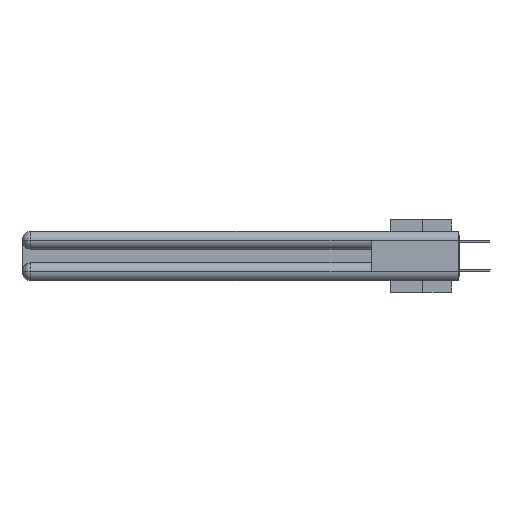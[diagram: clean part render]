
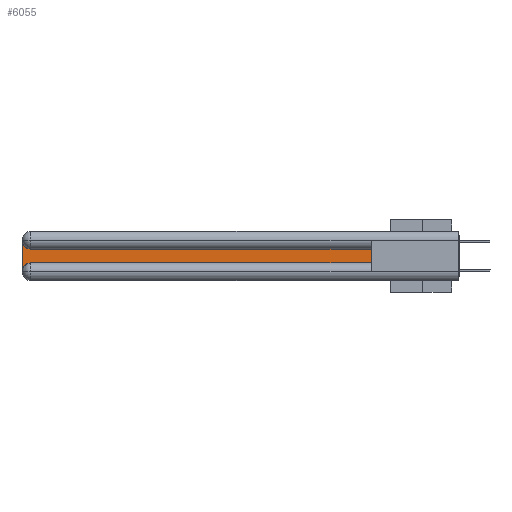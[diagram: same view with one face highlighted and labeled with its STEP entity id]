
A CAD part, left-side view. The second image highlights one B-rep face of the part: STEP entity #6055.
In plain terms, the highlighted planar face has unit normal (-1, 0, 0).
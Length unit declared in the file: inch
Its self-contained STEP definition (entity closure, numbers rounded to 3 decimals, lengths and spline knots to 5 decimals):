
#115 = CARTESIAN_POINT ( 'NONE',  ( 0.075, 3., -0.1225 ) ) ;
#227 = CIRCLE ( 'NONE', #17963, 0.06 ) ;
#2074 = VERTEX_POINT ( 'NONE', #14930 ) ;
#3064 = LINE ( 'NONE', #18936, #39791 ) ;
#4405 = CARTESIAN_POINT ( 'NONE',  ( 0.075, 3., -0.2775 ) ) ;
#5194 = PLANE ( 'NONE',  #10513 ) ;
#5320 = CARTESIAN_POINT ( 'NONE',  ( 0.075, 0.6, -0.2175 ) ) ;
#5392 = EDGE_LOOP ( 'NONE', ( #15820, #13317, #13856, #15604, #39094, #19469 ) ) ;
#6055 = ADVANCED_FACE ( 'NONE', ( #27139 ), #5194, .F. ) ;
#6175 = DIRECTION ( 'NONE',  ( 1., 0., 0. ) ) ;
#9086 = CARTESIAN_POINT ( 'NONE',  ( 0.075, 0.6, -0.1225 ) ) ;
#9203 = CARTESIAN_POINT ( 'NONE',  ( 0.075, 2.94, -0.0625 ) ) ;
#9964 = LINE ( 'NONE', #5320, #36097 ) ;
#10513 = AXIS2_PLACEMENT_3D ( 'NONE', #115, #6175, #31109 ) ;
#11548 = AXIS2_PLACEMENT_3D ( 'NONE', #35712, #32727, #23700 ) ;
#12958 = VECTOR ( 'NONE', #15416, 39.37008 ) ;
#13014 = VERTEX_POINT ( 'NONE', #26994 ) ;
#13314 = VERTEX_POINT ( 'NONE', #35372 ) ;
#13317 = ORIENTED_EDGE ( 'NONE', *, *, #33289, .T. ) ;
#13856 = ORIENTED_EDGE ( 'NONE', *, *, #18891, .T. ) ;
#14930 = CARTESIAN_POINT ( 'NONE',  ( 0.075, 2.94, -0.2175 ) ) ;
#15144 = LINE ( 'NONE', #26406, #33915 ) ;
#15416 = DIRECTION ( 'NONE',  ( 0., 1., 0. ) ) ;
#15604 = ORIENTED_EDGE ( 'NONE', *, *, #34396, .T. ) ;
#15820 = ORIENTED_EDGE ( 'NONE', *, *, #38568, .T. ) ;
#17071 = CARTESIAN_POINT ( 'NONE',  ( 0.075, 2.94, -0.1225 ) ) ;
#17963 = AXIS2_PLACEMENT_3D ( 'NONE', #9203, #27300, #36989 ) ;
#18891 = EDGE_CURVE ( 'NONE', #13314, #24438, #15144, .T. ) ;
#18936 = CARTESIAN_POINT ( 'NONE',  ( 0.075, 0.6, -0.2175 ) ) ;
#19469 = ORIENTED_EDGE ( 'NONE', *, *, #34130, .T. ) ;
#22025 = DIRECTION ( 'NONE',  ( 0., 0., 1. ) ) ;
#23086 = EDGE_CURVE ( 'NONE', #2074, #13014, #9964, .T. ) ;
#23700 = DIRECTION ( 'NONE',  ( 0., 0., -1. ) ) ;
#24438 = VERTEX_POINT ( 'NONE', #4405 ) ;
#25274 = VERTEX_POINT ( 'NONE', #17071 ) ;
#26406 = CARTESIAN_POINT ( 'NONE',  ( 0.075, 3., -0.2175 ) ) ;
#26994 = CARTESIAN_POINT ( 'NONE',  ( 0.075, 0.6, -0.2175 ) ) ;
#27010 = LINE ( 'NONE', #9086, #12958 ) ;
#27139 = FACE_OUTER_BOUND ( 'NONE', #5392, .T. ) ;
#27300 = DIRECTION ( 'NONE',  ( 1., 0., 0. ) ) ;
#28104 = VERTEX_POINT ( 'NONE', #30978 ) ;
#30118 = DIRECTION ( 'NONE',  ( 0., -1., 0. ) ) ;
#30978 = CARTESIAN_POINT ( 'NONE',  ( 0.075, 0.6, -0.1225 ) ) ;
#31109 = DIRECTION ( 'NONE',  ( 0., 0., -1. ) ) ;
#32727 = DIRECTION ( 'NONE',  ( 1., 0., 0. ) ) ;
#33289 = EDGE_CURVE ( 'NONE', #25274, #13314, #227, .T. ) ;
#33915 = VECTOR ( 'NONE', #38281, 39.37008 ) ;
#34130 = EDGE_CURVE ( 'NONE', #13014, #28104, #3064, .T. ) ;
#34396 = EDGE_CURVE ( 'NONE', #24438, #2074, #39422, .T. ) ;
#35372 = CARTESIAN_POINT ( 'NONE',  ( 0.075, 3., -0.0625 ) ) ;
#35712 = CARTESIAN_POINT ( 'NONE',  ( 0.075, 2.94, -0.2775 ) ) ;
#36097 = VECTOR ( 'NONE', #30118, 39.37008 ) ;
#36989 = DIRECTION ( 'NONE',  ( 0., 0., -1. ) ) ;
#38281 = DIRECTION ( 'NONE',  ( 0., 0., -1. ) ) ;
#38568 = EDGE_CURVE ( 'NONE', #28104, #25274, #27010, .T. ) ;
#39094 = ORIENTED_EDGE ( 'NONE', *, *, #23086, .T. ) ;
#39422 = CIRCLE ( 'NONE', #11548, 0.06 ) ;
#39791 = VECTOR ( 'NONE', #22025, 39.37008 ) ;
